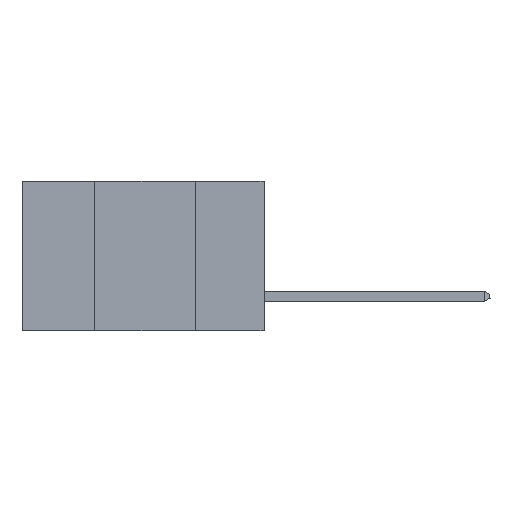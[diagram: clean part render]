
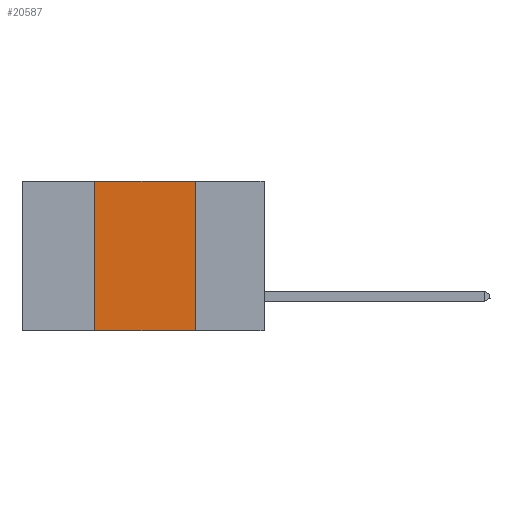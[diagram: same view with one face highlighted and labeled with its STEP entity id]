
A CAD part, left-side view. The second image highlights one B-rep face of the part: STEP entity #20587.
In plain terms, the highlighted planar face has unit normal (-1, 0, 0).
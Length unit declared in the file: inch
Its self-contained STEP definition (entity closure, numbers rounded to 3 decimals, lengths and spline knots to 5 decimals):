
#289 = CARTESIAN_POINT ( 'NONE',  ( 0., 0.17, 0. ) ) ;
#476 = ORIENTED_EDGE ( 'NONE', *, *, #14031, .F. ) ;
#865 = CARTESIAN_POINT ( 'NONE',  ( 0., 0.6, 0. ) ) ;
#2662 = DIRECTION ( 'NONE',  ( 0., 0., -1. ) ) ;
#3553 = VERTEX_POINT ( 'NONE', #7110 ) ;
#5762 = LINE ( 'NONE', #7105, #6017 ) ;
#6017 = VECTOR ( 'NONE', #20815, 39.37008 ) ;
#6096 = FACE_OUTER_BOUND ( 'NONE', #19774, .T. ) ;
#6114 = EDGE_CURVE ( 'NONE', #3553, #21149, #17580, .T. ) ;
#6257 = VECTOR ( 'NONE', #7673, 39.37008 ) ;
#7105 = CARTESIAN_POINT ( 'NONE',  ( 0., 0.42, 0. ) ) ;
#7110 = CARTESIAN_POINT ( 'NONE',  ( 0., 0.42, -0.37 ) ) ;
#7673 = DIRECTION ( 'NONE',  ( 0., -1., 0. ) ) ;
#7966 = CARTESIAN_POINT ( 'NONE',  ( 0., 0.6, -0.37 ) ) ;
#9320 = VERTEX_POINT ( 'NONE', #289 ) ;
#9503 = EDGE_CURVE ( 'NONE', #13384, #9320, #9717, .T. ) ;
#9625 = ORIENTED_EDGE ( 'NONE', *, *, #6114, .T. ) ;
#9717 = LINE ( 'NONE', #865, #6257 ) ;
#9735 = CARTESIAN_POINT ( 'NONE',  ( 0., 0.42, 0. ) ) ;
#11189 = CARTESIAN_POINT ( 'NONE',  ( 0., 0.6, 0. ) ) ;
#11739 = DIRECTION ( 'NONE',  ( 0., 0., -1. ) ) ;
#12909 = DIRECTION ( 'NONE',  ( 0., -1., 0. ) ) ;
#13384 = VERTEX_POINT ( 'NONE', #9735 ) ;
#13606 = CARTESIAN_POINT ( 'NONE',  ( 0., 0.17, 0. ) ) ;
#14031 = EDGE_CURVE ( 'NONE', #9320, #21149, #17128, .T. ) ;
#15806 = CARTESIAN_POINT ( 'NONE',  ( 0., 0.17, -0.37 ) ) ;
#16218 = PLANE ( 'NONE',  #17018 ) ;
#16369 = DIRECTION ( 'NONE',  ( 1., 0., 0. ) ) ;
#16928 = EDGE_CURVE ( 'NONE', #3553, #13384, #5762, .T. ) ;
#17018 = AXIS2_PLACEMENT_3D ( 'NONE', #11189, #16369, #2662 ) ;
#17128 = LINE ( 'NONE', #13606, #18740 ) ;
#17580 = LINE ( 'NONE', #7966, #20516 ) ;
#18740 = VECTOR ( 'NONE', #11739, 39.37008 ) ;
#18856 = ORIENTED_EDGE ( 'NONE', *, *, #16928, .F. ) ;
#19774 = EDGE_LOOP ( 'NONE', ( #476, #21733, #18856, #9625 ) ) ;
#20516 = VECTOR ( 'NONE', #12909, 39.37008 ) ;
#20587 = ADVANCED_FACE ( 'NONE', ( #6096 ), #16218, .F. ) ;
#20815 = DIRECTION ( 'NONE',  ( 0., 0., 1. ) ) ;
#21149 = VERTEX_POINT ( 'NONE', #15806 ) ;
#21733 = ORIENTED_EDGE ( 'NONE', *, *, #9503, .F. ) ;
